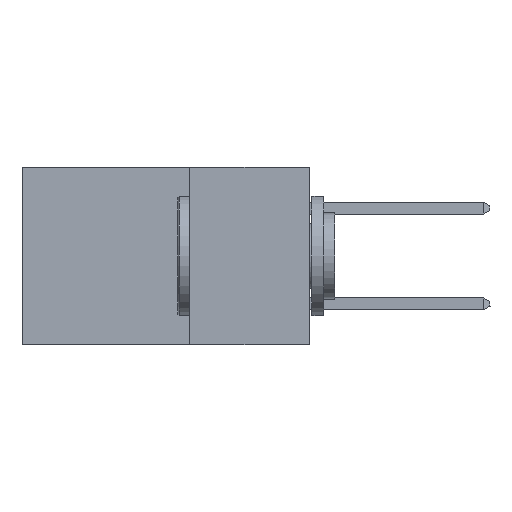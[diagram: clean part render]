
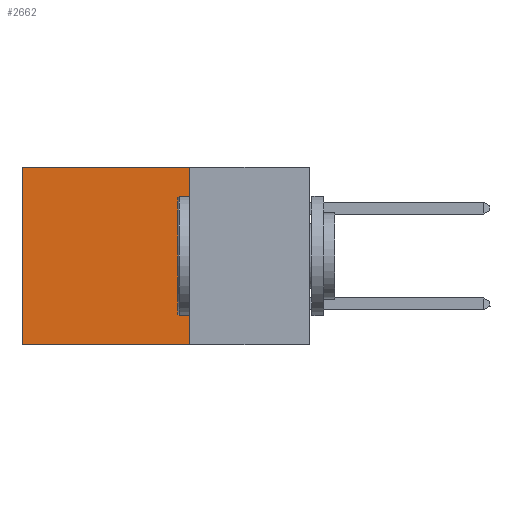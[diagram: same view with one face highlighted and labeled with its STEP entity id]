
A CAD part, left-side view. The second image highlights one B-rep face of the part: STEP entity #2662.
In plain terms, the highlighted planar face has unit normal (-1, 0, 0).
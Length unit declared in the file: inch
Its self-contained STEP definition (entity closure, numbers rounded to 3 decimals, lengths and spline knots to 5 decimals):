
#1874 = ORIENTED_EDGE ( 'NONE', *, *, #10402, .T. ) ;
#2662 = ADVANCED_FACE ( 'NONE', ( #9018 ), #5063, .F. ) ;
#3687 = LINE ( 'NONE', #18400, #19518 ) ;
#3803 = EDGE_CURVE ( 'NONE', #12024, #4170, #3687, .T. ) ;
#4170 = VERTEX_POINT ( 'NONE', #21833 ) ;
#4916 = DIRECTION ( 'NONE',  ( 0., 1., 0. ) ) ;
#5063 = PLANE ( 'NONE',  #17860 ) ;
#5933 = VECTOR ( 'NONE', #21463, 39.37008 ) ;
#6208 = CARTESIAN_POINT ( 'NONE',  ( 0.2875, 0.25, 0. ) ) ;
#7350 = LINE ( 'NONE', #19203, #5933 ) ;
#7367 = CARTESIAN_POINT ( 'NONE',  ( 0.2875, 0.25, 0. ) ) ;
#7711 = EDGE_LOOP ( 'NONE', ( #1874, #20707, #27903, #14376 ) ) ;
#8732 = DIRECTION ( 'NONE',  ( 0., 1., 0. ) ) ;
#8737 = VERTEX_POINT ( 'NONE', #20397 ) ;
#8841 = CARTESIAN_POINT ( 'NONE',  ( 0.2875, 0.6, 0. ) ) ;
#9018 = FACE_OUTER_BOUND ( 'NONE', #7711, .T. ) ;
#10402 = EDGE_CURVE ( 'NONE', #8737, #4170, #18292, .T. ) ;
#11899 = DIRECTION ( 'NONE',  ( 0., 0., -1. ) ) ;
#12024 = VERTEX_POINT ( 'NONE', #19261 ) ;
#12336 = VECTOR ( 'NONE', #26770, 39.37008 ) ;
#14077 = LINE ( 'NONE', #19911, #24596 ) ;
#14376 = ORIENTED_EDGE ( 'NONE', *, *, #25897, .T. ) ;
#17860 = AXIS2_PLACEMENT_3D ( 'NONE', #7367, #25345, #11899 ) ;
#18292 = LINE ( 'NONE', #8841, #12336 ) ;
#18400 = CARTESIAN_POINT ( 'NONE',  ( 0.2875, 0.25, -0.37 ) ) ;
#19203 = CARTESIAN_POINT ( 'NONE',  ( 0.2875, 0.25, 0. ) ) ;
#19261 = CARTESIAN_POINT ( 'NONE',  ( 0.2875, 0.25, -0.37 ) ) ;
#19518 = VECTOR ( 'NONE', #4916, 39.37008 ) ;
#19911 = CARTESIAN_POINT ( 'NONE',  ( 0.2875, 0.25, 0. ) ) ;
#20397 = CARTESIAN_POINT ( 'NONE',  ( 0.2875, 0.6, 0. ) ) ;
#20707 = ORIENTED_EDGE ( 'NONE', *, *, #3803, .F. ) ;
#21250 = VERTEX_POINT ( 'NONE', #6208 ) ;
#21463 = DIRECTION ( 'NONE',  ( 0., 0., -1. ) ) ;
#21833 = CARTESIAN_POINT ( 'NONE',  ( 0.2875, 0.6, -0.37 ) ) ;
#24596 = VECTOR ( 'NONE', #8732, 39.37008 ) ;
#25345 = DIRECTION ( 'NONE',  ( 1., 0., 0. ) ) ;
#25897 = EDGE_CURVE ( 'NONE', #21250, #8737, #14077, .T. ) ;
#26376 = EDGE_CURVE ( 'NONE', #21250, #12024, #7350, .T. ) ;
#26770 = DIRECTION ( 'NONE',  ( 0., 0., -1. ) ) ;
#27903 = ORIENTED_EDGE ( 'NONE', *, *, #26376, .F. ) ;
